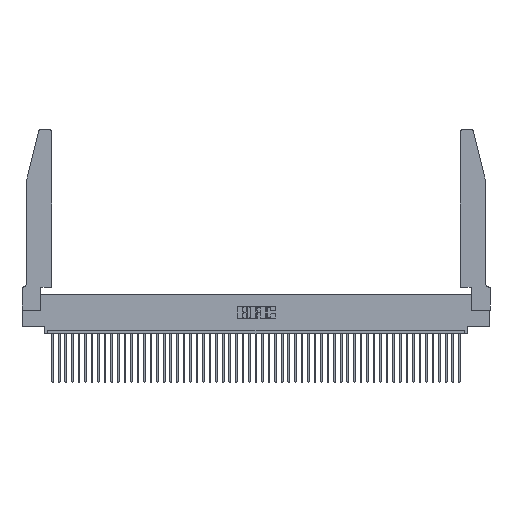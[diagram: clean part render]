
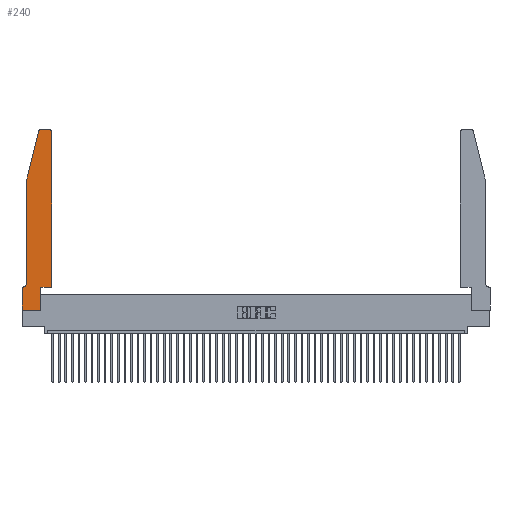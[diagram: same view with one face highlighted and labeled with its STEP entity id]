
A CAD part, top view. The second image highlights one B-rep face of the part: STEP entity #240.
In plain terms, the highlighted planar face has unit normal (0, 0, 1).
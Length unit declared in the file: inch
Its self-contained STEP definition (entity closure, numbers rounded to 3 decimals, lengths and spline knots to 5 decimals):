
#152 = AXIS2_PLACEMENT_3D ( 'NONE', #31821, #8817, #17106 ) ;
#240 = ADVANCED_FACE ( 'NONE', ( #18856 ), #40929, .T. ) ;
#1098 = CARTESIAN_POINT ( 'NONE',  ( 0.2865, 0.35, 0.37 ) ) ;
#1435 = LINE ( 'NONE', #45859, #3281 ) ;
#2190 = CARTESIAN_POINT ( 'NONE',  ( 0., 0.35, 0.37 ) ) ;
#2421 = ORIENTED_EDGE ( 'NONE', *, *, #33262, .T. ) ;
#2629 = EDGE_CURVE ( 'NONE', #3096, #20707, #11028, .T. ) ;
#3096 = VERTEX_POINT ( 'NONE', #25067 ) ;
#3270 = ORIENTED_EDGE ( 'NONE', *, *, #34476, .T. ) ;
#3281 = VECTOR ( 'NONE', #26188, 39.37008 ) ;
#3579 = CARTESIAN_POINT ( 'NONE',  ( 0.0755, 0.35, 0.37 ) ) ;
#3789 = VECTOR ( 'NONE', #10977, 39.37008 ) ;
#4642 = CARTESIAN_POINT ( 'NONE',  ( 0.0755, 2., 0.37 ) ) ;
#4726 = ORIENTED_EDGE ( 'NONE', *, *, #45581, .T. ) ;
#4908 = LINE ( 'NONE', #15368, #3789 ) ;
#5064 = LINE ( 'NONE', #31404, #15387 ) ;
#5901 = CARTESIAN_POINT ( 'NONE',  ( 0.0055, 0.35, 0.37 ) ) ;
#6543 = DIRECTION ( 'NONE',  ( 0., 0., 1. ) ) ;
#6895 = ORIENTED_EDGE ( 'NONE', *, *, #40691, .T. ) ;
#7785 = VERTEX_POINT ( 'NONE', #37399 ) ;
#8003 = AXIS2_PLACEMENT_3D ( 'NONE', #35732, #43250, #19870 ) ;
#8027 = LINE ( 'NONE', #15998, #46976 ) ;
#8547 = VERTEX_POINT ( 'NONE', #48580 ) ;
#8817 = DIRECTION ( 'NONE',  ( 0., 0., -1. ) ) ;
#9363 = CIRCLE ( 'NONE', #152, 0.07 ) ;
#10019 = EDGE_CURVE ( 'NONE', #15248, #7785, #32036, .T. ) ;
#10977 = DIRECTION ( 'NONE',  ( -0.239, -0.971, 0. ) ) ;
#11028 = LINE ( 'NONE', #36053, #21237 ) ;
#12431 = CIRCLE ( 'NONE', #8003, 0.03 ) ;
#12630 = DIRECTION ( 'NONE',  ( 1., 0., 0. ) ) ;
#12779 = DIRECTION ( 'NONE',  ( 0., 1., 0. ) ) ;
#12935 = CARTESIAN_POINT ( 'NONE',  ( 0.25487, 2.72718, 0.37 ) ) ;
#14640 = VERTEX_POINT ( 'NONE', #27238 ) ;
#14806 = VECTOR ( 'NONE', #33256, 39.37008 ) ;
#14934 = EDGE_CURVE ( 'NONE', #19006, #14640, #44918, .T. ) ;
#15224 = AXIS2_PLACEMENT_3D ( 'NONE', #18047, #45130, #43858 ) ;
#15248 = VERTEX_POINT ( 'NONE', #36747 ) ;
#15368 = CARTESIAN_POINT ( 'NONE',  ( 0.0755, 2., 0.37 ) ) ;
#15387 = VECTOR ( 'NONE', #12630, 39.37008 ) ;
#15747 = EDGE_CURVE ( 'NONE', #31385, #29652, #9363, .T. ) ;
#15998 = CARTESIAN_POINT ( 'NONE',  ( 0.4505, 0.35, 0.37 ) ) ;
#16482 = LINE ( 'NONE', #1098, #14806 ) ;
#17014 = DIRECTION ( 'NONE',  ( 1., 0., 0. ) ) ;
#17106 = DIRECTION ( 'NONE',  ( -1., 0., 0. ) ) ;
#17235 = VERTEX_POINT ( 'NONE', #4642 ) ;
#17285 = DIRECTION ( 'NONE',  ( 1., 0., 0. ) ) ;
#18047 = CARTESIAN_POINT ( 'NONE',  ( 0.4205, 2.72, 0.37 ) ) ;
#18856 = FACE_OUTER_BOUND ( 'NONE', #20784, .T. ) ;
#19006 = VERTEX_POINT ( 'NONE', #49203 ) ;
#19870 = DIRECTION ( 'NONE',  ( 1., 0., 0. ) ) ;
#20285 = EDGE_CURVE ( 'NONE', #8547, #15248, #16482, .T. ) ;
#20707 = VERTEX_POINT ( 'NONE', #29137 ) ;
#20784 = EDGE_LOOP ( 'NONE', ( #2421, #25756, #3270, #23420, #43537, #4726, #42087, #23548, #21463, #26563, #6895, #35657 ) ) ;
#20990 = EDGE_CURVE ( 'NONE', #17235, #31385, #1435, .T. ) ;
#21237 = VECTOR ( 'NONE', #47568, 39.37008 ) ;
#21463 = ORIENTED_EDGE ( 'NONE', *, *, #20285, .T. ) ;
#21758 = VERTEX_POINT ( 'NONE', #44676 ) ;
#22449 = VECTOR ( 'NONE', #34112, 39.37008 ) ;
#23420 = ORIENTED_EDGE ( 'NONE', *, *, #20990, .T. ) ;
#23548 = ORIENTED_EDGE ( 'NONE', *, *, #31023, .T. ) ;
#23659 = VECTOR ( 'NONE', #17014, 39.37008 ) ;
#24737 = EDGE_CURVE ( 'NONE', #21758, #32433, #12431, .T. ) ;
#25067 = CARTESIAN_POINT ( 'NONE',  ( 0., 0.35, 0.37 ) ) ;
#25756 = ORIENTED_EDGE ( 'NONE', *, *, #24737, .T. ) ;
#26188 = DIRECTION ( 'NONE',  ( 0., -1., 0. ) ) ;
#26309 = DIRECTION ( 'NONE',  ( -1., 0., 0. ) ) ;
#26563 = ORIENTED_EDGE ( 'NONE', *, *, #10019, .T. ) ;
#27238 = CARTESIAN_POINT ( 'NONE',  ( 0.4205, 2.75, 0.37 ) ) ;
#29137 = CARTESIAN_POINT ( 'NONE',  ( 0., 0., 0.37 ) ) ;
#29652 = VERTEX_POINT ( 'NONE', #5901 ) ;
#31023 = EDGE_CURVE ( 'NONE', #20707, #8547, #5064, .T. ) ;
#31385 = VERTEX_POINT ( 'NONE', #35694 ) ;
#31404 = CARTESIAN_POINT ( 'NONE',  ( 0., 0., 0.37 ) ) ;
#31821 = CARTESIAN_POINT ( 'NONE',  ( 0.0055, 0.42, 0.37 ) ) ;
#32036 = LINE ( 'NONE', #43965, #23659 ) ;
#32433 = VERTEX_POINT ( 'NONE', #12935 ) ;
#33110 = AXIS2_PLACEMENT_3D ( 'NONE', #2190, #6543, #17285 ) ;
#33256 = DIRECTION ( 'NONE',  ( 0., 1., 0. ) ) ;
#33262 = EDGE_CURVE ( 'NONE', #14640, #21758, #39226, .T. ) ;
#34112 = DIRECTION ( 'NONE',  ( -1., 0., 0. ) ) ;
#34389 = LINE ( 'NONE', #3579, #22449 ) ;
#34476 = EDGE_CURVE ( 'NONE', #32433, #17235, #4908, .T. ) ;
#35657 = ORIENTED_EDGE ( 'NONE', *, *, #14934, .T. ) ;
#35694 = CARTESIAN_POINT ( 'NONE',  ( 0.0755, 0.42, 0.37 ) ) ;
#35732 = CARTESIAN_POINT ( 'NONE',  ( 0.284, 2.72, 0.37 ) ) ;
#36053 = CARTESIAN_POINT ( 'NONE',  ( 0., 0., 0.37 ) ) ;
#36747 = CARTESIAN_POINT ( 'NONE',  ( 0.2865, 0.35, 0.37 ) ) ;
#37399 = CARTESIAN_POINT ( 'NONE',  ( 0.4505, 0.35, 0.37 ) ) ;
#39226 = LINE ( 'NONE', #41195, #42805 ) ;
#40691 = EDGE_CURVE ( 'NONE', #7785, #19006, #8027, .T. ) ;
#40929 = PLANE ( 'NONE',  #33110 ) ;
#41195 = CARTESIAN_POINT ( 'NONE',  ( 0.2605, 2.75, 0.37 ) ) ;
#42087 = ORIENTED_EDGE ( 'NONE', *, *, #2629, .T. ) ;
#42805 = VECTOR ( 'NONE', #26309, 39.37008 ) ;
#43250 = DIRECTION ( 'NONE',  ( 0., 0., 1. ) ) ;
#43537 = ORIENTED_EDGE ( 'NONE', *, *, #15747, .T. ) ;
#43858 = DIRECTION ( 'NONE',  ( 1., 0., 0. ) ) ;
#43965 = CARTESIAN_POINT ( 'NONE',  ( 0.4505, 0.35, 0.37 ) ) ;
#44676 = CARTESIAN_POINT ( 'NONE',  ( 0.284, 2.75, 0.37 ) ) ;
#44918 = CIRCLE ( 'NONE', #15224, 0.03 ) ;
#45130 = DIRECTION ( 'NONE',  ( 0., 0., 1. ) ) ;
#45581 = EDGE_CURVE ( 'NONE', #29652, #3096, #34389, .T. ) ;
#45859 = CARTESIAN_POINT ( 'NONE',  ( 0.0755, 2., 0.37 ) ) ;
#46976 = VECTOR ( 'NONE', #12779, 39.37008 ) ;
#47568 = DIRECTION ( 'NONE',  ( 0., -1., 0. ) ) ;
#48580 = CARTESIAN_POINT ( 'NONE',  ( 0.2865, 0., 0.37 ) ) ;
#49203 = CARTESIAN_POINT ( 'NONE',  ( 0.4505, 2.72, 0.37 ) ) ;
